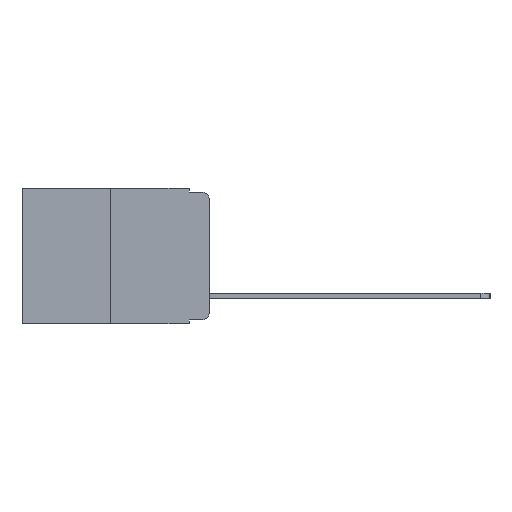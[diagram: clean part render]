
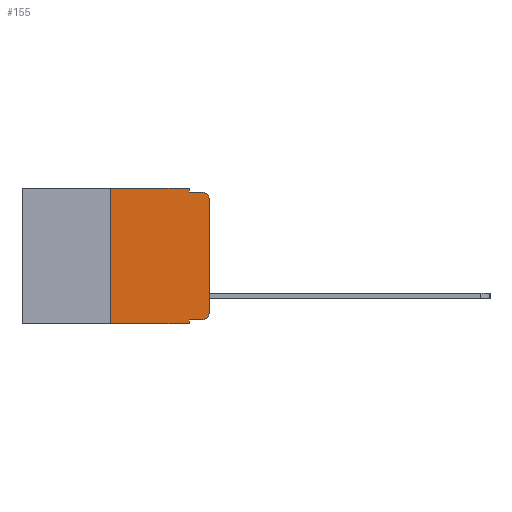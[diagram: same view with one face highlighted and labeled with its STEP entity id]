
A CAD part, left-side view. The second image highlights one B-rep face of the part: STEP entity #155.
In plain terms, the highlighted planar face has unit normal (-1, 0, 0).
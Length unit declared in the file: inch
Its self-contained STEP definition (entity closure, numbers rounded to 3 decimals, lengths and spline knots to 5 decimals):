
#129 = ORIENTED_EDGE ( 'NONE', *, *, #10480, .F. ) ;
#155 = ADVANCED_FACE ( 'NONE', ( #8117 ), #9995, .F. ) ;
#533 = VERTEX_POINT ( 'NONE', #2756 ) ;
#1029 = VERTEX_POINT ( 'NONE', #10228 ) ;
#1060 = VERTEX_POINT ( 'NONE', #3590 ) ;
#1078 = ORIENTED_EDGE ( 'NONE', *, *, #6611, .T. ) ;
#1168 = CIRCLE ( 'NONE', #9234, 0.02 ) ;
#1421 = DIRECTION ( 'NONE',  ( 0., 0., 1. ) ) ;
#1696 = VECTOR ( 'NONE', #9949, 39.37008 ) ;
#1703 = CARTESIAN_POINT ( 'NONE',  ( 0., 0.473, -0.343 ) ) ;
#1706 = CARTESIAN_POINT ( 'NONE',  ( 0., 0.473, 0. ) ) ;
#1833 = ORIENTED_EDGE ( 'NONE', *, *, #11181, .T. ) ;
#2137 = CARTESIAN_POINT ( 'NONE',  ( 0., 0.473, 0. ) ) ;
#2277 = LINE ( 'NONE', #10051, #10466 ) ;
#2428 = VECTOR ( 'NONE', #5451, 39.37008 ) ;
#2569 = DIRECTION ( 'NONE',  ( -1., 0., 0. ) ) ;
#2756 = CARTESIAN_POINT ( 'NONE',  ( 0., 0.02, -0.333 ) ) ;
#2764 = VERTEX_POINT ( 'NONE', #10871 ) ;
#3430 = AXIS2_PLACEMENT_3D ( 'NONE', #9284, #2569, #10369 ) ;
#3590 = CARTESIAN_POINT ( 'NONE',  ( 0., 0.051, -0.01 ) ) ;
#3600 = VERTEX_POINT ( 'NONE', #12491 ) ;
#3839 = DIRECTION ( 'NONE',  ( 0., -1., 0. ) ) ;
#3882 = VECTOR ( 'NONE', #1421, 39.37008 ) ;
#3960 = ORIENTED_EDGE ( 'NONE', *, *, #9750, .F. ) ;
#4439 = DIRECTION ( 'NONE',  ( 0., 0., -1. ) ) ;
#4540 = LINE ( 'NONE', #14131, #1696 ) ;
#4716 = ORIENTED_EDGE ( 'NONE', *, *, #4928, .F. ) ;
#4877 = LINE ( 'NONE', #9472, #14025 ) ;
#4888 = DIRECTION ( 'NONE',  ( 0., -1., 0. ) ) ;
#4928 = EDGE_CURVE ( 'NONE', #8299, #8182, #5215, .T. ) ;
#5106 = CARTESIAN_POINT ( 'NONE',  ( 0., 0.02, -0.01 ) ) ;
#5215 = LINE ( 'NONE', #1706, #2428 ) ;
#5451 = DIRECTION ( 'NONE',  ( 0., -1., 0. ) ) ;
#5752 = VECTOR ( 'NONE', #4888, 39.37008 ) ;
#6064 = VERTEX_POINT ( 'NONE', #5106 ) ;
#6071 = DIRECTION ( 'NONE',  ( 1., 0., 0. ) ) ;
#6216 = VECTOR ( 'NONE', #11618, 39.37008 ) ;
#6602 = DIRECTION ( 'NONE',  ( 0., 0., -1. ) ) ;
#6611 = EDGE_CURVE ( 'NONE', #533, #3600, #1168, .T. ) ;
#6778 = LINE ( 'NONE', #1703, #9533 ) ;
#7079 = VERTEX_POINT ( 'NONE', #7111 ) ;
#7111 = CARTESIAN_POINT ( 'NONE',  ( 0., 0.051, -0.343 ) ) ;
#7253 = ORIENTED_EDGE ( 'NONE', *, *, #9025, .F. ) ;
#7332 = AXIS2_PLACEMENT_3D ( 'NONE', #2137, #6071, #4439 ) ;
#7435 = ORIENTED_EDGE ( 'NONE', *, *, #8233, .F. ) ;
#7454 = EDGE_CURVE ( 'NONE', #2764, #533, #11152, .T. ) ;
#8117 = FACE_OUTER_BOUND ( 'NONE', #12266, .T. ) ;
#8164 = ORIENTED_EDGE ( 'NONE', *, *, #7454, .T. ) ;
#8182 = VERTEX_POINT ( 'NONE', #8809 ) ;
#8233 = EDGE_CURVE ( 'NONE', #2764, #7079, #2277, .T. ) ;
#8299 = VERTEX_POINT ( 'NONE', #10242 ) ;
#8809 = CARTESIAN_POINT ( 'NONE',  ( 0., 0.051, 0. ) ) ;
#9025 = EDGE_CURVE ( 'NONE', #11622, #8299, #4877, .T. ) ;
#9234 = AXIS2_PLACEMENT_3D ( 'NONE', #11993, #12611, #11617 ) ;
#9284 = CARTESIAN_POINT ( 'NONE',  ( 0., 0.02, -0.03 ) ) ;
#9381 = LINE ( 'NONE', #10565, #6216 ) ;
#9472 = CARTESIAN_POINT ( 'NONE',  ( 0., 0.25, 0. ) ) ;
#9533 = VECTOR ( 'NONE', #3839, 39.37008 ) ;
#9710 = CIRCLE ( 'NONE', #3430, 0.02 ) ;
#9750 = EDGE_CURVE ( 'NONE', #8182, #1060, #4540, .T. ) ;
#9949 = DIRECTION ( 'NONE',  ( 0., 0., -1. ) ) ;
#9995 = PLANE ( 'NONE',  #7332 ) ;
#10051 = CARTESIAN_POINT ( 'NONE',  ( 0., 0.051, 0. ) ) ;
#10228 = CARTESIAN_POINT ( 'NONE',  ( 0., 0., -0.03 ) ) ;
#10242 = CARTESIAN_POINT ( 'NONE',  ( 0., 0.25, 0. ) ) ;
#10310 = CARTESIAN_POINT ( 'NONE',  ( 0., 0., 0. ) ) ;
#10369 = DIRECTION ( 'NONE',  ( 0., 0., -1. ) ) ;
#10466 = VECTOR ( 'NONE', #6602, 39.37008 ) ;
#10480 = EDGE_CURVE ( 'NONE', #1060, #6064, #9381, .T. ) ;
#10565 = CARTESIAN_POINT ( 'NONE',  ( 0., 0.051, -0.01 ) ) ;
#10573 = ORIENTED_EDGE ( 'NONE', *, *, #13712, .T. ) ;
#10821 = CARTESIAN_POINT ( 'NONE',  ( 0., 0.25, -0.343 ) ) ;
#10871 = CARTESIAN_POINT ( 'NONE',  ( 0., 0.051, -0.333 ) ) ;
#11152 = LINE ( 'NONE', #11634, #5752 ) ;
#11181 = EDGE_CURVE ( 'NONE', #1029, #6064, #9710, .T. ) ;
#11617 = DIRECTION ( 'NONE',  ( 0., 0., -1. ) ) ;
#11618 = DIRECTION ( 'NONE',  ( 0., -1., 0. ) ) ;
#11622 = VERTEX_POINT ( 'NONE', #10821 ) ;
#11634 = CARTESIAN_POINT ( 'NONE',  ( 0., 0.051, -0.333 ) ) ;
#11898 = EDGE_CURVE ( 'NONE', #3600, #1029, #13046, .T. ) ;
#11993 = CARTESIAN_POINT ( 'NONE',  ( 0., 0.02, -0.313 ) ) ;
#12266 = EDGE_LOOP ( 'NONE', ( #13019, #1833, #129, #3960, #4716, #7253, #10573, #7435, #8164, #1078 ) ) ;
#12491 = CARTESIAN_POINT ( 'NONE',  ( 0., 0., -0.313 ) ) ;
#12611 = DIRECTION ( 'NONE',  ( -1., 0., 0. ) ) ;
#12653 = DIRECTION ( 'NONE',  ( 0., 0., 1. ) ) ;
#13019 = ORIENTED_EDGE ( 'NONE', *, *, #11898, .T. ) ;
#13046 = LINE ( 'NONE', #10310, #3882 ) ;
#13712 = EDGE_CURVE ( 'NONE', #11622, #7079, #6778, .T. ) ;
#14025 = VECTOR ( 'NONE', #12653, 39.37008 ) ;
#14131 = CARTESIAN_POINT ( 'NONE',  ( 0., 0.051, 0. ) ) ;
